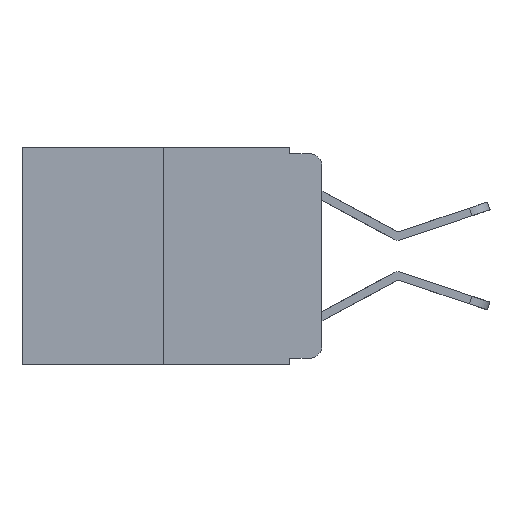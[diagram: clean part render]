
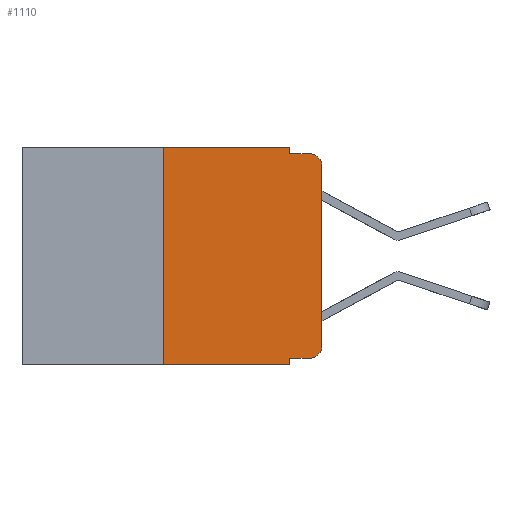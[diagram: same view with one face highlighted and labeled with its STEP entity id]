
A CAD part, left-side view. The second image highlights one B-rep face of the part: STEP entity #1110.
In plain terms, the highlighted planar face has unit normal (-1, 0, 0).
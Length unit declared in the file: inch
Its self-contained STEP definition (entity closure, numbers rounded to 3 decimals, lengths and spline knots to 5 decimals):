
#81 = EDGE_CURVE ( 'NONE', #20994, #15450, #16218, .T. ) ;
#792 = ORIENTED_EDGE ( 'NONE', *, *, #16545, .T. ) ;
#974 = LINE ( 'NONE', #7822, #17766 ) ;
#1110 = ADVANCED_FACE ( 'NONE', ( #3248 ), #7496, .F. ) ;
#1261 = EDGE_CURVE ( 'NONE', #5892, #15450, #14191, .T. ) ;
#1382 = CARTESIAN_POINT ( 'NONE',  ( 0., 0.051, 0. ) ) ;
#1554 = VERTEX_POINT ( 'NONE', #15004 ) ;
#1833 = CARTESIAN_POINT ( 'NONE',  ( 0., 0.051, -0.01 ) ) ;
#2386 = DIRECTION ( 'NONE',  ( 1., 0., 0. ) ) ;
#2459 = VECTOR ( 'NONE', #4709, 39.37008 ) ;
#2526 = DIRECTION ( 'NONE',  ( 0., 0., -1. ) ) ;
#2782 = CARTESIAN_POINT ( 'NONE',  ( 0., 0.02, -0.03 ) ) ;
#2784 = AXIS2_PLACEMENT_3D ( 'NONE', #7413, #2386, #13427 ) ;
#3248 = FACE_OUTER_BOUND ( 'NONE', #9455, .T. ) ;
#4479 = DIRECTION ( 'NONE',  ( -1., 0., 0. ) ) ;
#4555 = DIRECTION ( 'NONE',  ( -1., 0., 0. ) ) ;
#4709 = DIRECTION ( 'NONE',  ( 0., 0., -1. ) ) ;
#4770 = CARTESIAN_POINT ( 'NONE',  ( 0., 0.051, -0.333 ) ) ;
#4962 = CARTESIAN_POINT ( 'NONE',  ( 0., 0.051, -0.333 ) ) ;
#5892 = VERTEX_POINT ( 'NONE', #19423 ) ;
#6116 = VERTEX_POINT ( 'NONE', #12167 ) ;
#6252 = CARTESIAN_POINT ( 'NONE',  ( 0., 0.051, -0.01 ) ) ;
#6697 = DIRECTION ( 'NONE',  ( 0., -1., 0. ) ) ;
#7351 = ORIENTED_EDGE ( 'NONE', *, *, #13107, .T. ) ;
#7371 = VECTOR ( 'NONE', #8644, 39.37008 ) ;
#7413 = CARTESIAN_POINT ( 'NONE',  ( 0., 0.473, 0. ) ) ;
#7496 = PLANE ( 'NONE',  #2784 ) ;
#7822 = CARTESIAN_POINT ( 'NONE',  ( 0., 0.473, -0.343 ) ) ;
#8302 = AXIS2_PLACEMENT_3D ( 'NONE', #2782, #4479, #2526 ) ;
#8644 = DIRECTION ( 'NONE',  ( 0., 0., -1. ) ) ;
#8823 = CARTESIAN_POINT ( 'NONE',  ( 0., 0.02, -0.333 ) ) ;
#8876 = LINE ( 'NONE', #15810, #17366 ) ;
#9140 = VERTEX_POINT ( 'NONE', #4770 ) ;
#9455 = EDGE_LOOP ( 'NONE', ( #20220, #10094, #12166, #9870, #14667, #20780, #792, #9630, #10637, #7351 ) ) ;
#9485 = CARTESIAN_POINT ( 'NONE',  ( 0., 0.02, -0.01 ) ) ;
#9630 = ORIENTED_EDGE ( 'NONE', *, *, #10923, .F. ) ;
#9837 = EDGE_CURVE ( 'NONE', #9140, #13510, #19151, .T. ) ;
#9870 = ORIENTED_EDGE ( 'NONE', *, *, #10514, .F. ) ;
#9970 = VERTEX_POINT ( 'NONE', #16507 ) ;
#10094 = ORIENTED_EDGE ( 'NONE', *, *, #1261, .T. ) ;
#10514 = EDGE_CURVE ( 'NONE', #16194, #20994, #19100, .T. ) ;
#10598 = DIRECTION ( 'NONE',  ( 0., 0., 1. ) ) ;
#10637 = ORIENTED_EDGE ( 'NONE', *, *, #9837, .T. ) ;
#10824 = EDGE_CURVE ( 'NONE', #9970, #16194, #8876, .T. ) ;
#10923 = EDGE_CURVE ( 'NONE', #9140, #12630, #15433, .T. ) ;
#11043 = DIRECTION ( 'NONE',  ( 0., -1., 0. ) ) ;
#11427 = DIRECTION ( 'NONE',  ( 0., -1., 0. ) ) ;
#11444 = CARTESIAN_POINT ( 'NONE',  ( 0., 0.051, 0. ) ) ;
#11985 = VECTOR ( 'NONE', #6697, 39.37008 ) ;
#12166 = ORIENTED_EDGE ( 'NONE', *, *, #81, .F. ) ;
#12167 = CARTESIAN_POINT ( 'NONE',  ( 0., 0.25, -0.343 ) ) ;
#12454 = CARTESIAN_POINT ( 'NONE',  ( 0., 0.25, 0. ) ) ;
#12573 = VECTOR ( 'NONE', #10598, 39.37008 ) ;
#12630 = VERTEX_POINT ( 'NONE', #17845 ) ;
#13107 = EDGE_CURVE ( 'NONE', #13510, #1554, #17064, .T. ) ;
#13427 = DIRECTION ( 'NONE',  ( 0., 0., -1. ) ) ;
#13510 = VERTEX_POINT ( 'NONE', #8823 ) ;
#14002 = VECTOR ( 'NONE', #11427, 39.37008 ) ;
#14071 = EDGE_CURVE ( 'NONE', #6116, #9970, #19234, .T. ) ;
#14191 = CIRCLE ( 'NONE', #8302, 0.02 ) ;
#14275 = CARTESIAN_POINT ( 'NONE',  ( 0., 0.02, -0.313 ) ) ;
#14667 = ORIENTED_EDGE ( 'NONE', *, *, #10824, .F. ) ;
#15004 = CARTESIAN_POINT ( 'NONE',  ( 0., 0., -0.313 ) ) ;
#15433 = LINE ( 'NONE', #1382, #2459 ) ;
#15450 = VERTEX_POINT ( 'NONE', #9485 ) ;
#15608 = AXIS2_PLACEMENT_3D ( 'NONE', #14275, #4555, #15881 ) ;
#15810 = CARTESIAN_POINT ( 'NONE',  ( 0., 0.473, 0. ) ) ;
#15881 = DIRECTION ( 'NONE',  ( 0., 0., -1. ) ) ;
#16194 = VERTEX_POINT ( 'NONE', #11444 ) ;
#16218 = LINE ( 'NONE', #6252, #11985 ) ;
#16507 = CARTESIAN_POINT ( 'NONE',  ( 0., 0.25, 0. ) ) ;
#16545 = EDGE_CURVE ( 'NONE', #6116, #12630, #974, .T. ) ;
#16984 = EDGE_CURVE ( 'NONE', #1554, #5892, #17253, .T. ) ;
#17064 = CIRCLE ( 'NONE', #15608, 0.02 ) ;
#17253 = LINE ( 'NONE', #18494, #12573 ) ;
#17366 = VECTOR ( 'NONE', #11043, 39.37008 ) ;
#17766 = VECTOR ( 'NONE', #20542, 39.37008 ) ;
#17845 = CARTESIAN_POINT ( 'NONE',  ( 0., 0.051, -0.343 ) ) ;
#18494 = CARTESIAN_POINT ( 'NONE',  ( 0., 0., 0. ) ) ;
#18706 = DIRECTION ( 'NONE',  ( 0., 0., 1. ) ) ;
#18728 = VECTOR ( 'NONE', #18706, 39.37008 ) ;
#19100 = LINE ( 'NONE', #19713, #7371 ) ;
#19151 = LINE ( 'NONE', #4962, #14002 ) ;
#19234 = LINE ( 'NONE', #12454, #18728 ) ;
#19423 = CARTESIAN_POINT ( 'NONE',  ( 0., 0., -0.03 ) ) ;
#19713 = CARTESIAN_POINT ( 'NONE',  ( 0., 0.051, 0. ) ) ;
#20220 = ORIENTED_EDGE ( 'NONE', *, *, #16984, .T. ) ;
#20542 = DIRECTION ( 'NONE',  ( 0., -1., 0. ) ) ;
#20780 = ORIENTED_EDGE ( 'NONE', *, *, #14071, .F. ) ;
#20994 = VERTEX_POINT ( 'NONE', #1833 ) ;
